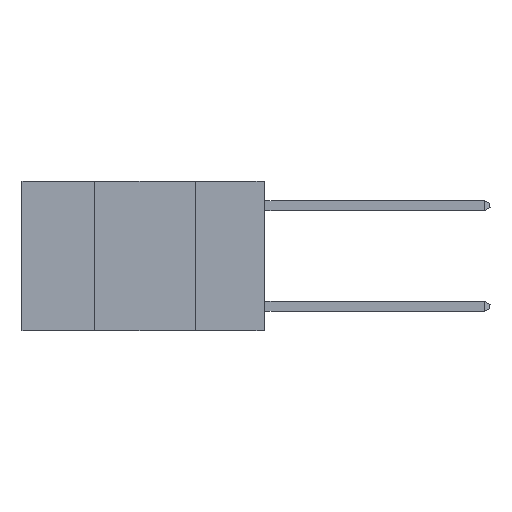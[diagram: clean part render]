
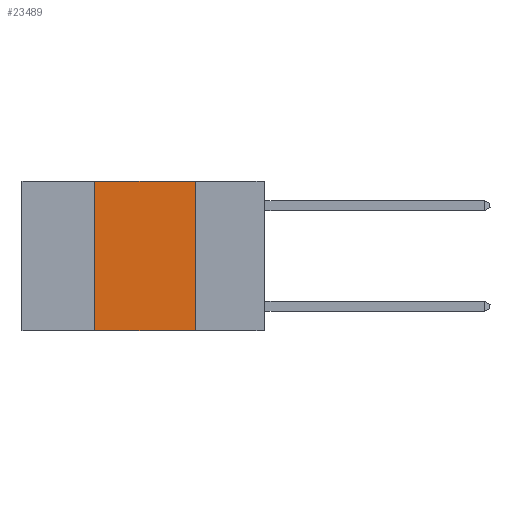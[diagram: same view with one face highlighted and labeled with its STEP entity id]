
A CAD part, left-side view. The second image highlights one B-rep face of the part: STEP entity #23489.
In plain terms, the highlighted planar face has unit normal (-1, 0, 0).
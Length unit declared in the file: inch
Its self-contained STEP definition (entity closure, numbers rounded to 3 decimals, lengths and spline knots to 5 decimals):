
#1623 = VECTOR ( 'NONE', #8888, 39.37008 ) ;
#1829 = CARTESIAN_POINT ( 'NONE',  ( 0., 0.42, 0. ) ) ;
#2047 = DIRECTION ( 'NONE',  ( 0., -1., 0. ) ) ;
#2915 = CARTESIAN_POINT ( 'NONE',  ( 0., 0.42, 0. ) ) ;
#4164 = CARTESIAN_POINT ( 'NONE',  ( 0., 0.6, 0. ) ) ;
#5220 = DIRECTION ( 'NONE',  ( 0., 0., 1. ) ) ;
#5515 = CARTESIAN_POINT ( 'NONE',  ( 0., 0.42, -0.37 ) ) ;
#6597 = CARTESIAN_POINT ( 'NONE',  ( 0., 0.17, -0.37 ) ) ;
#8158 = ORIENTED_EDGE ( 'NONE', *, *, #27823, .F. ) ;
#8255 = CARTESIAN_POINT ( 'NONE',  ( 0., 0.17, 0. ) ) ;
#8888 = DIRECTION ( 'NONE',  ( 0., 0., -1. ) ) ;
#10050 = VERTEX_POINT ( 'NONE', #8255 ) ;
#10260 = CARTESIAN_POINT ( 'NONE',  ( 0., 0.6, 0. ) ) ;
#10343 = DIRECTION ( 'NONE',  ( 0., 0., -1. ) ) ;
#10552 = CARTESIAN_POINT ( 'NONE',  ( 0., 0.6, -0.37 ) ) ;
#12792 = EDGE_CURVE ( 'NONE', #26770, #23578, #20834, .T. ) ;
#13339 = VECTOR ( 'NONE', #2047, 39.37008 ) ;
#13511 = ORIENTED_EDGE ( 'NONE', *, *, #21220, .F. ) ;
#14479 = EDGE_LOOP ( 'NONE', ( #8158, #13511, #27063, #16377 ) ) ;
#14977 = FACE_OUTER_BOUND ( 'NONE', #14479, .T. ) ;
#15190 = LINE ( 'NONE', #10552, #13339 ) ;
#15378 = AXIS2_PLACEMENT_3D ( 'NONE', #4164, #27986, #10343 ) ;
#15756 = VECTOR ( 'NONE', #5220, 39.37008 ) ;
#16377 = ORIENTED_EDGE ( 'NONE', *, *, #17560, .T. ) ;
#16637 = LINE ( 'NONE', #10260, #22677 ) ;
#17560 = EDGE_CURVE ( 'NONE', #26770, #18613, #15190, .T. ) ;
#18613 = VERTEX_POINT ( 'NONE', #6597 ) ;
#20834 = LINE ( 'NONE', #2915, #15756 ) ;
#21220 = EDGE_CURVE ( 'NONE', #23578, #10050, #16637, .T. ) ;
#21775 = CARTESIAN_POINT ( 'NONE',  ( 0., 0.17, 0. ) ) ;
#22677 = VECTOR ( 'NONE', #25738, 39.37008 ) ;
#23489 = ADVANCED_FACE ( 'NONE', ( #14977 ), #23936, .F. ) ;
#23578 = VERTEX_POINT ( 'NONE', #1829 ) ;
#23936 = PLANE ( 'NONE',  #15378 ) ;
#24360 = LINE ( 'NONE', #21775, #1623 ) ;
#25738 = DIRECTION ( 'NONE',  ( 0., -1., 0. ) ) ;
#26770 = VERTEX_POINT ( 'NONE', #5515 ) ;
#27063 = ORIENTED_EDGE ( 'NONE', *, *, #12792, .F. ) ;
#27823 = EDGE_CURVE ( 'NONE', #10050, #18613, #24360, .T. ) ;
#27986 = DIRECTION ( 'NONE',  ( 1., 0., 0. ) ) ;
